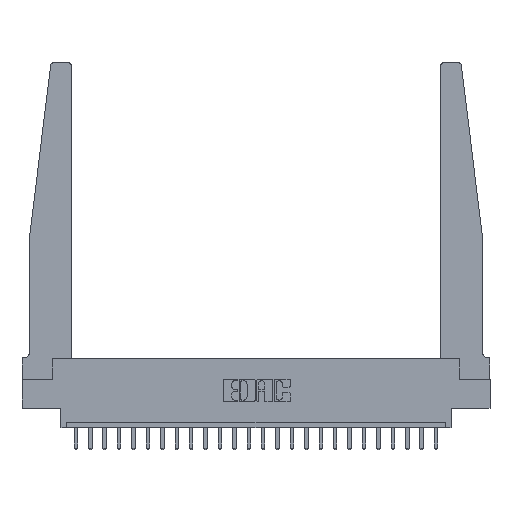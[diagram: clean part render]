
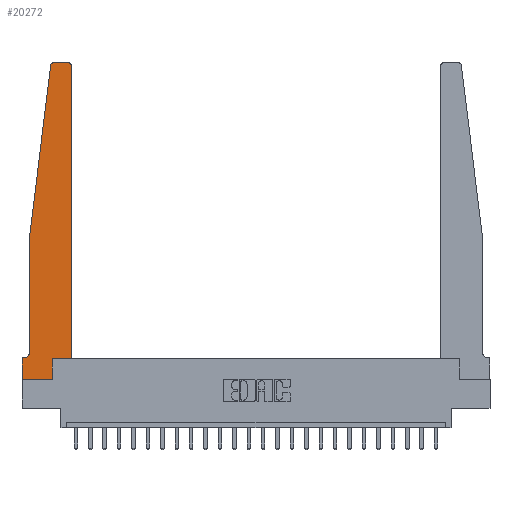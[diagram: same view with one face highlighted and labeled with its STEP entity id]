
A CAD part, top view. The second image highlights one B-rep face of the part: STEP entity #20272.
In plain terms, the highlighted planar face has unit normal (0, 0, 1).
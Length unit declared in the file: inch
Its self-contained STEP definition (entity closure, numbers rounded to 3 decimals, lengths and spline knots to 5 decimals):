
#20 = CARTESIAN_POINT ( 'NONE',  ( 0.065, 0.1875, 0.37 ) ) ;
#81 = DIRECTION ( 'NONE',  ( 1., 0., 0. ) ) ;
#132 = ORIENTED_EDGE ( 'NONE', *, *, #16861, .T. ) ;
#509 = ORIENTED_EDGE ( 'NONE', *, *, #14546, .T. ) ;
#879 = DIRECTION ( 'NONE',  ( -1., 0., 0. ) ) ;
#1631 = LINE ( 'NONE', #12788, #22010 ) ;
#1685 = CIRCLE ( 'NONE', #18953, 0.03 ) ;
#1790 = AXIS2_PLACEMENT_3D ( 'NONE', #10117, #17443, #22983 ) ;
#1797 = CARTESIAN_POINT ( 'NONE',  ( 0.015, 0.1875, 0.37 ) ) ;
#1926 = VERTEX_POINT ( 'NONE', #13175 ) ;
#1933 = LINE ( 'NONE', #20, #6603 ) ;
#2109 = VERTEX_POINT ( 'NONE', #1797 ) ;
#2178 = VERTEX_POINT ( 'NONE', #14397 ) ;
#2195 = CARTESIAN_POINT ( 'NONE',  ( 0.065, 1.25, 0.37 ) ) ;
#2364 = ORIENTED_EDGE ( 'NONE', *, *, #19894, .T. ) ;
#2805 = PLANE ( 'NONE',  #1790 ) ;
#2946 = DIRECTION ( 'NONE',  ( 1., 0., 0. ) ) ;
#3092 = VERTEX_POINT ( 'NONE', #23109 ) ;
#3625 = ORIENTED_EDGE ( 'NONE', *, *, #11598, .T. ) ;
#3643 = CIRCLE ( 'NONE', #4010, 0.03 ) ;
#3695 = VERTEX_POINT ( 'NONE', #20293 ) ;
#4010 = AXIS2_PLACEMENT_3D ( 'NONE', #12685, #12561, #81 ) ;
#4394 = ORIENTED_EDGE ( 'NONE', *, *, #7259, .T. ) ;
#4477 = DIRECTION ( 'NONE',  ( -0.122, -0.992, 0. ) ) ;
#4849 = DIRECTION ( 'NONE',  ( -1., 0., 0. ) ) ;
#6392 = VERTEX_POINT ( 'NONE', #18888 ) ;
#6450 = CARTESIAN_POINT ( 'NONE',  ( 0.425, 0.18, 0.37 ) ) ;
#6603 = VECTOR ( 'NONE', #16943, 39.37008 ) ;
#6998 = ORIENTED_EDGE ( 'NONE', *, *, #15682, .T. ) ;
#7146 = DIRECTION ( 'NONE',  ( 0., 1., 0. ) ) ;
#7259 = EDGE_CURVE ( 'NONE', #22751, #3695, #20843, .T. ) ;
#7381 = DIRECTION ( 'NONE',  ( 0., 0., 1. ) ) ;
#7810 = ORIENTED_EDGE ( 'NONE', *, *, #16795, .T. ) ;
#7990 = VECTOR ( 'NONE', #8087, 39.37008 ) ;
#7999 = VERTEX_POINT ( 'NONE', #13078 ) ;
#8087 = DIRECTION ( 'NONE',  ( 1., 0., 0. ) ) ;
#8090 = ORIENTED_EDGE ( 'NONE', *, *, #12376, .T. ) ;
#8104 = LINE ( 'NONE', #23127, #18254 ) ;
#8205 = CARTESIAN_POINT ( 'NONE',  ( 0.25, 2.75, 0.37 ) ) ;
#8841 = DIRECTION ( 'NONE',  ( 1., 0., 0. ) ) ;
#8963 = CARTESIAN_POINT ( 'NONE',  ( 0.065, 1.25, 0.37 ) ) ;
#9631 = ORIENTED_EDGE ( 'NONE', *, *, #10787, .T. ) ;
#9885 = FACE_OUTER_BOUND ( 'NONE', #10545, .T. ) ;
#10117 = CARTESIAN_POINT ( 'NONE',  ( 0., 0.1875, 0.37 ) ) ;
#10194 = LINE ( 'NONE', #22943, #15367 ) ;
#10504 = EDGE_CURVE ( 'NONE', #23065, #7999, #12323, .T. ) ;
#10545 = EDGE_LOOP ( 'NONE', ( #9631, #7810, #8090, #132, #21456, #23466, #509, #4394, #3625, #2364, #11584, #6998 ) ) ;
#10787 = EDGE_CURVE ( 'NONE', #15650, #3092, #11703, .T. ) ;
#11002 = LINE ( 'NONE', #8963, #22440 ) ;
#11025 = CARTESIAN_POINT ( 'NONE',  ( 0.065, 0.2375, 0.37 ) ) ;
#11584 = ORIENTED_EDGE ( 'NONE', *, *, #10504, .T. ) ;
#11598 = EDGE_CURVE ( 'NONE', #3695, #17417, #10194, .T. ) ;
#11703 = LINE ( 'NONE', #8205, #20755 ) ;
#11805 = CARTESIAN_POINT ( 'NONE',  ( 0.2605, 0.18, 0.37 ) ) ;
#12323 = LINE ( 'NONE', #17841, #16871 ) ;
#12376 = EDGE_CURVE ( 'NONE', #6392, #1926, #18662, .T. ) ;
#12532 = EDGE_CURVE ( 'NONE', #18101, #2109, #19264, .T. ) ;
#12553 = DIRECTION ( 'NONE',  ( 0., -1., 0. ) ) ;
#12561 = DIRECTION ( 'NONE',  ( 0., 0., 1. ) ) ;
#12685 = CARTESIAN_POINT ( 'NONE',  ( 0.27653, 2.72, 0.37 ) ) ;
#12775 = EDGE_CURVE ( 'NONE', #2109, #2178, #1933, .T. ) ;
#12788 = CARTESIAN_POINT ( 'NONE',  ( 0., 0., 0.37 ) ) ;
#13078 = CARTESIAN_POINT ( 'NONE',  ( 0.425, 2.72, 0.37 ) ) ;
#13175 = CARTESIAN_POINT ( 'NONE',  ( 0.065, 1.25, 0.37 ) ) ;
#13319 = DIRECTION ( 'NONE',  ( 0., 1., 0. ) ) ;
#14397 = CARTESIAN_POINT ( 'NONE',  ( 0., 0.1875, 0.37 ) ) ;
#14546 = EDGE_CURVE ( 'NONE', #2178, #22751, #1631, .T. ) ;
#15367 = VECTOR ( 'NONE', #13319, 39.37008 ) ;
#15650 = VERTEX_POINT ( 'NONE', #20042 ) ;
#15682 = EDGE_CURVE ( 'NONE', #7999, #15650, #1685, .T. ) ;
#16278 = CARTESIAN_POINT ( 'NONE',  ( 0.395, 2.72, 0.37 ) ) ;
#16285 = DIRECTION ( 'NONE',  ( 0., -1., 0. ) ) ;
#16795 = EDGE_CURVE ( 'NONE', #3092, #6392, #3643, .T. ) ;
#16861 = EDGE_CURVE ( 'NONE', #1926, #18101, #11002, .T. ) ;
#16871 = VECTOR ( 'NONE', #7146, 39.37008 ) ;
#16943 = DIRECTION ( 'NONE',  ( -1., 0., 0. ) ) ;
#17223 = CARTESIAN_POINT ( 'NONE',  ( 0., 0., 0.37 ) ) ;
#17331 = DIRECTION ( 'NONE',  ( 0., 0., -1. ) ) ;
#17417 = VERTEX_POINT ( 'NONE', #11805 ) ;
#17443 = DIRECTION ( 'NONE',  ( 0., 0., 1. ) ) ;
#17561 = CARTESIAN_POINT ( 'NONE',  ( 0.015, 0.2375, 0.37 ) ) ;
#17841 = CARTESIAN_POINT ( 'NONE',  ( 0.425, 0.18, 0.37 ) ) ;
#18101 = VERTEX_POINT ( 'NONE', #11025 ) ;
#18254 = VECTOR ( 'NONE', #2946, 39.37008 ) ;
#18662 = LINE ( 'NONE', #2195, #21563 ) ;
#18888 = CARTESIAN_POINT ( 'NONE',  ( 0.24675, 2.72367, 0.37 ) ) ;
#18953 = AXIS2_PLACEMENT_3D ( 'NONE', #16278, #7381, #8841 ) ;
#19264 = CIRCLE ( 'NONE', #21947, 0.05 ) ;
#19894 = EDGE_CURVE ( 'NONE', #17417, #23065, #8104, .T. ) ;
#20042 = CARTESIAN_POINT ( 'NONE',  ( 0.395, 2.75, 0.37 ) ) ;
#20272 = ADVANCED_FACE ( 'NONE', ( #9885 ), #2805, .T. ) ;
#20293 = CARTESIAN_POINT ( 'NONE',  ( 0.2605, 0., 0.37 ) ) ;
#20755 = VECTOR ( 'NONE', #4849, 39.37008 ) ;
#20843 = LINE ( 'NONE', #17223, #7990 ) ;
#21456 = ORIENTED_EDGE ( 'NONE', *, *, #12532, .T. ) ;
#21563 = VECTOR ( 'NONE', #4477, 39.37008 ) ;
#21630 = CARTESIAN_POINT ( 'NONE',  ( 0., 0., 0.37 ) ) ;
#21947 = AXIS2_PLACEMENT_3D ( 'NONE', #17561, #17331, #879 ) ;
#22010 = VECTOR ( 'NONE', #12553, 39.37008 ) ;
#22440 = VECTOR ( 'NONE', #16285, 39.37008 ) ;
#22751 = VERTEX_POINT ( 'NONE', #21630 ) ;
#22943 = CARTESIAN_POINT ( 'NONE',  ( 0.2605, 0.18, 0.37 ) ) ;
#22983 = DIRECTION ( 'NONE',  ( 1., 0., 0. ) ) ;
#23065 = VERTEX_POINT ( 'NONE', #6450 ) ;
#23109 = CARTESIAN_POINT ( 'NONE',  ( 0.27653, 2.75, 0.37 ) ) ;
#23127 = CARTESIAN_POINT ( 'NONE',  ( 0.425, 0.18, 0.37 ) ) ;
#23466 = ORIENTED_EDGE ( 'NONE', *, *, #12775, .T. ) ;
